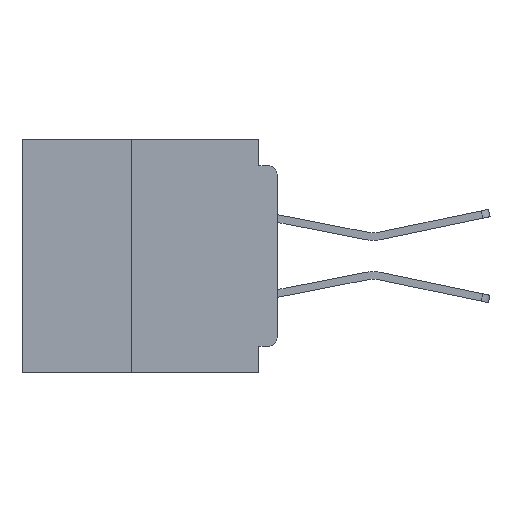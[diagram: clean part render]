
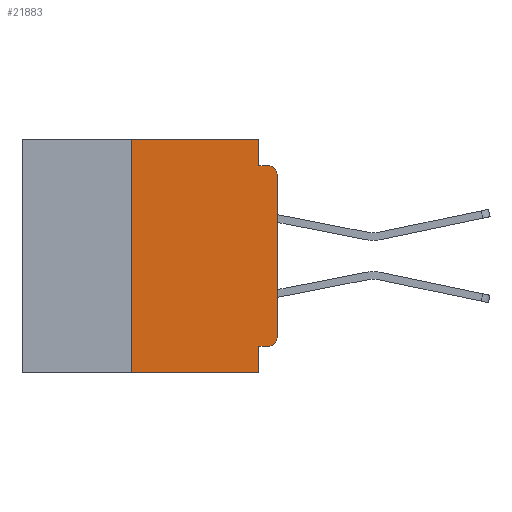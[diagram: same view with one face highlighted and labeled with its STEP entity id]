
A CAD part, left-side view. The second image highlights one B-rep face of the part: STEP entity #21883.
In plain terms, the highlighted planar face has unit normal (-1, 0, 0).
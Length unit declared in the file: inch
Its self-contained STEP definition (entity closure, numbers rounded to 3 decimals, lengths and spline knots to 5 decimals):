
#39 = CARTESIAN_POINT ( 'NONE',  ( 0., 0.031, -0.045 ) ) ;
#2232 = DIRECTION ( 'NONE',  ( 1., 0., 0. ) ) ;
#2820 = DIRECTION ( 'NONE',  ( -1., 0., 0. ) ) ;
#3299 = CARTESIAN_POINT ( 'NONE',  ( 0., 0.25, -0.4 ) ) ;
#3905 = DIRECTION ( 'NONE',  ( 0., -1., 0. ) ) ;
#4104 = CARTESIAN_POINT ( 'NONE',  ( 0., 0.015, -0.045 ) ) ;
#5493 = VECTOR ( 'NONE', #41223, 39.37008 ) ;
#6222 = CARTESIAN_POINT ( 'NONE',  ( 0., 0.031, 0. ) ) ;
#7496 = CARTESIAN_POINT ( 'NONE',  ( 0., 0., -0.355 ) ) ;
#8258 = CARTESIAN_POINT ( 'NONE',  ( 0., 0., -0.06 ) ) ;
#8289 = EDGE_CURVE ( 'NONE', #11951, #48852, #34611, .T. ) ;
#8330 = AXIS2_PLACEMENT_3D ( 'NONE', #26436, #2820, #30398 ) ;
#8331 = DIRECTION ( 'NONE',  ( 0., 0., -1. ) ) ;
#9209 = EDGE_CURVE ( 'NONE', #46297, #36347, #43818, .T. ) ;
#9453 = EDGE_CURVE ( 'NONE', #48852, #31422, #11707, .T. ) ;
#9645 = CARTESIAN_POINT ( 'NONE',  ( 0., 0., -0.045 ) ) ;
#10515 = VERTEX_POINT ( 'NONE', #4104 ) ;
#11268 = VERTEX_POINT ( 'NONE', #32481 ) ;
#11707 = LINE ( 'NONE', #17700, #21020 ) ;
#11951 = VERTEX_POINT ( 'NONE', #37436 ) ;
#13932 = EDGE_CURVE ( 'NONE', #31422, #10515, #34145, .T. ) ;
#14741 = LINE ( 'NONE', #38945, #34477 ) ;
#16002 = VERTEX_POINT ( 'NONE', #6222 ) ;
#16083 = VECTOR ( 'NONE', #27260, 39.37008 ) ;
#16152 = CARTESIAN_POINT ( 'NONE',  ( 0., 0.031, -0.4 ) ) ;
#16357 = CARTESIAN_POINT ( 'NONE',  ( 0., 0.015, -0.06 ) ) ;
#17336 = LINE ( 'NONE', #23323, #16083 ) ;
#17700 = CARTESIAN_POINT ( 'NONE',  ( 0., 0., 0. ) ) ;
#19126 = EDGE_CURVE ( 'NONE', #29211, #36347, #17336, .T. ) ;
#19303 = ORIENTED_EDGE ( 'NONE', *, *, #19126, .T. ) ;
#19351 = EDGE_CURVE ( 'NONE', #29211, #11268, #46863, .T. ) ;
#19586 = ORIENTED_EDGE ( 'NONE', *, *, #9209, .F. ) ;
#19626 = CARTESIAN_POINT ( 'NONE',  ( 0., 0.437, 0. ) ) ;
#20351 = DIRECTION ( 'NONE',  ( 0., 0., -1. ) ) ;
#20478 = LINE ( 'NONE', #19626, #50625 ) ;
#20701 = CARTESIAN_POINT ( 'NONE',  ( 0., 0., -0.34 ) ) ;
#21020 = VECTOR ( 'NONE', #49181, 39.37008 ) ;
#21679 = VECTOR ( 'NONE', #8331, 39.37008 ) ;
#21883 = ADVANCED_FACE ( 'NONE', ( #23011 ), #49417, .F. ) ;
#21930 = CARTESIAN_POINT ( 'NONE',  ( 0., 0.437, 0. ) ) ;
#21984 = EDGE_LOOP ( 'NONE', ( #48604, #41899, #47880, #29837, #49249, #37364, #19303, #19586, #27404, #44039 ) ) ;
#22832 = VERTEX_POINT ( 'NONE', #39 ) ;
#23011 = FACE_OUTER_BOUND ( 'NONE', #21984, .T. ) ;
#23323 = CARTESIAN_POINT ( 'NONE',  ( 0., 0.437, -0.4 ) ) ;
#26436 = CARTESIAN_POINT ( 'NONE',  ( 0., 0.015, -0.34 ) ) ;
#27260 = DIRECTION ( 'NONE',  ( 0., -1., 0. ) ) ;
#27404 = ORIENTED_EDGE ( 'NONE', *, *, #46455, .F. ) ;
#29211 = VERTEX_POINT ( 'NONE', #3299 ) ;
#29811 = DIRECTION ( 'NONE',  ( 0., 0., -1. ) ) ;
#29837 = ORIENTED_EDGE ( 'NONE', *, *, #31905, .F. ) ;
#30398 = DIRECTION ( 'NONE',  ( 0., 0., -1. ) ) ;
#30405 = VECTOR ( 'NONE', #42864, 39.37008 ) ;
#30704 = EDGE_CURVE ( 'NONE', #11268, #16002, #20478, .T. ) ;
#30958 = AXIS2_PLACEMENT_3D ( 'NONE', #21930, #2232, #29811 ) ;
#31422 = VERTEX_POINT ( 'NONE', #8258 ) ;
#31628 = LINE ( 'NONE', #7496, #30405 ) ;
#31905 = EDGE_CURVE ( 'NONE', #16002, #22832, #14741, .T. ) ;
#32481 = CARTESIAN_POINT ( 'NONE',  ( 0., 0.25, 0. ) ) ;
#34145 = CIRCLE ( 'NONE', #45906, 0.015 ) ;
#34477 = VECTOR ( 'NONE', #42894, 39.37008 ) ;
#34611 = CIRCLE ( 'NONE', #8330, 0.015 ) ;
#35175 = VECTOR ( 'NONE', #36525, 39.37008 ) ;
#36347 = VERTEX_POINT ( 'NONE', #38879 ) ;
#36525 = DIRECTION ( 'NONE',  ( 0., 0., 1. ) ) ;
#36978 = LINE ( 'NONE', #9645, #5493 ) ;
#37364 = ORIENTED_EDGE ( 'NONE', *, *, #19351, .F. ) ;
#37436 = CARTESIAN_POINT ( 'NONE',  ( 0., 0.015, -0.355 ) ) ;
#38879 = CARTESIAN_POINT ( 'NONE',  ( 0., 0.031, -0.4 ) ) ;
#38945 = CARTESIAN_POINT ( 'NONE',  ( 0., 0.031, 0. ) ) ;
#40512 = CARTESIAN_POINT ( 'NONE',  ( 0., 0.25, -0.4 ) ) ;
#41223 = DIRECTION ( 'NONE',  ( 0., -1., 0. ) ) ;
#41899 = ORIENTED_EDGE ( 'NONE', *, *, #13932, .T. ) ;
#42864 = DIRECTION ( 'NONE',  ( 0., 1., 0. ) ) ;
#42894 = DIRECTION ( 'NONE',  ( 0., 0., -1. ) ) ;
#43818 = LINE ( 'NONE', #16152, #21679 ) ;
#43912 = DIRECTION ( 'NONE',  ( -1., 0., 0. ) ) ;
#44039 = ORIENTED_EDGE ( 'NONE', *, *, #8289, .T. ) ;
#45805 = CARTESIAN_POINT ( 'NONE',  ( 0., 0.031, -0.355 ) ) ;
#45906 = AXIS2_PLACEMENT_3D ( 'NONE', #16357, #43912, #20351 ) ;
#46297 = VERTEX_POINT ( 'NONE', #45805 ) ;
#46455 = EDGE_CURVE ( 'NONE', #11951, #46297, #31628, .T. ) ;
#46863 = LINE ( 'NONE', #40512, #35175 ) ;
#47880 = ORIENTED_EDGE ( 'NONE', *, *, #48329, .F. ) ;
#48329 = EDGE_CURVE ( 'NONE', #22832, #10515, #36978, .T. ) ;
#48604 = ORIENTED_EDGE ( 'NONE', *, *, #9453, .T. ) ;
#48852 = VERTEX_POINT ( 'NONE', #20701 ) ;
#49181 = DIRECTION ( 'NONE',  ( 0., 0., 1. ) ) ;
#49249 = ORIENTED_EDGE ( 'NONE', *, *, #30704, .F. ) ;
#49417 = PLANE ( 'NONE',  #30958 ) ;
#50625 = VECTOR ( 'NONE', #3905, 39.37008 ) ;
